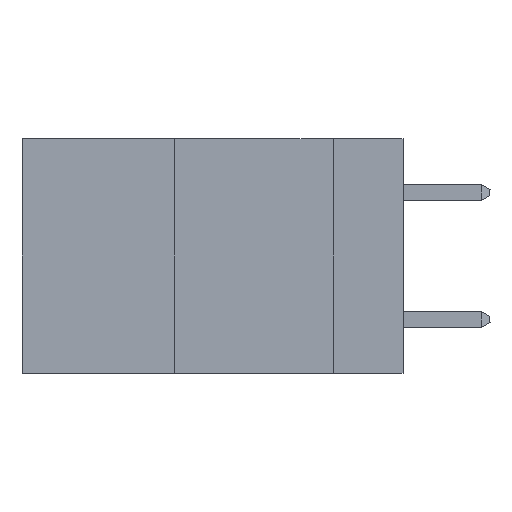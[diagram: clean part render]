
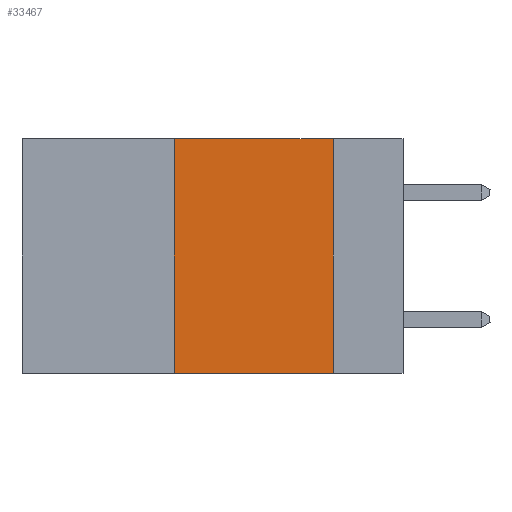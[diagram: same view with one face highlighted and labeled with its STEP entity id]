
A CAD part, left-side view. The second image highlights one B-rep face of the part: STEP entity #33467.
In plain terms, the highlighted planar face has unit normal (-1, 0, 0).
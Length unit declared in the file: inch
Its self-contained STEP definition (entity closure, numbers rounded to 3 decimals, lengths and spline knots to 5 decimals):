
#36 = LINE ( 'NONE', #2430, #28474 ) ;
#105 = CARTESIAN_POINT ( 'NONE',  ( 0., 0.6, 0. ) ) ;
#1692 = CARTESIAN_POINT ( 'NONE',  ( 0., 0.11, 0. ) ) ;
#1904 = CARTESIAN_POINT ( 'NONE',  ( 0., 0.36, 0. ) ) ;
#2132 = DIRECTION ( 'NONE',  ( 0., -1., 0. ) ) ;
#2430 = CARTESIAN_POINT ( 'NONE',  ( 0., 0.6, 0. ) ) ;
#2895 = LINE ( 'NONE', #7670, #15757 ) ;
#3388 = VERTEX_POINT ( 'NONE', #42145 ) ;
#4027 = CARTESIAN_POINT ( 'NONE',  ( 0., 0.11, 0. ) ) ;
#5326 = DIRECTION ( 'NONE',  ( 0., 0., -1. ) ) ;
#6865 = DIRECTION ( 'NONE',  ( 1., 0., 0. ) ) ;
#7670 = CARTESIAN_POINT ( 'NONE',  ( 0., 0.6, -0.37 ) ) ;
#9445 = AXIS2_PLACEMENT_3D ( 'NONE', #105, #6865, #28321 ) ;
#10412 = PLANE ( 'NONE',  #9445 ) ;
#12268 = CARTESIAN_POINT ( 'NONE',  ( 0., 0.36, -0.37 ) ) ;
#12745 = VERTEX_POINT ( 'NONE', #33302 ) ;
#14718 = VECTOR ( 'NONE', #23117, 39.37008 ) ;
#14863 = DIRECTION ( 'NONE',  ( 0., -1., 0. ) ) ;
#14953 = VERTEX_POINT ( 'NONE', #4027 ) ;
#15757 = VECTOR ( 'NONE', #14863, 39.37008 ) ;
#21216 = EDGE_CURVE ( 'NONE', #24954, #3388, #31441, .T. ) ;
#22024 = EDGE_CURVE ( 'NONE', #14953, #12745, #44828, .T. ) ;
#22376 = ORIENTED_EDGE ( 'NONE', *, *, #21216, .F. ) ;
#23117 = DIRECTION ( 'NONE',  ( 0., 0., 1. ) ) ;
#24367 = EDGE_LOOP ( 'NONE', ( #24810, #29117, #22376, #24652 ) ) ;
#24652 = ORIENTED_EDGE ( 'NONE', *, *, #41254, .T. ) ;
#24810 = ORIENTED_EDGE ( 'NONE', *, *, #22024, .F. ) ;
#24954 = VERTEX_POINT ( 'NONE', #12268 ) ;
#28321 = DIRECTION ( 'NONE',  ( 0., 0., -1. ) ) ;
#28474 = VECTOR ( 'NONE', #2132, 39.37008 ) ;
#29117 = ORIENTED_EDGE ( 'NONE', *, *, #31936, .F. ) ;
#31441 = LINE ( 'NONE', #1904, #14718 ) ;
#31936 = EDGE_CURVE ( 'NONE', #3388, #14953, #36, .T. ) ;
#33302 = CARTESIAN_POINT ( 'NONE',  ( 0., 0.11, -0.37 ) ) ;
#33467 = ADVANCED_FACE ( 'NONE', ( #41199 ), #10412, .F. ) ;
#41199 = FACE_OUTER_BOUND ( 'NONE', #24367, .T. ) ;
#41254 = EDGE_CURVE ( 'NONE', #24954, #12745, #2895, .T. ) ;
#42145 = CARTESIAN_POINT ( 'NONE',  ( 0., 0.36, 0. ) ) ;
#44828 = LINE ( 'NONE', #1692, #45932 ) ;
#45932 = VECTOR ( 'NONE', #5326, 39.37008 ) ;
